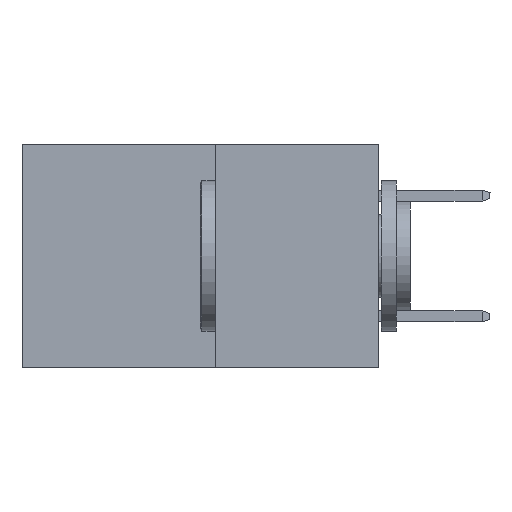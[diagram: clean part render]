
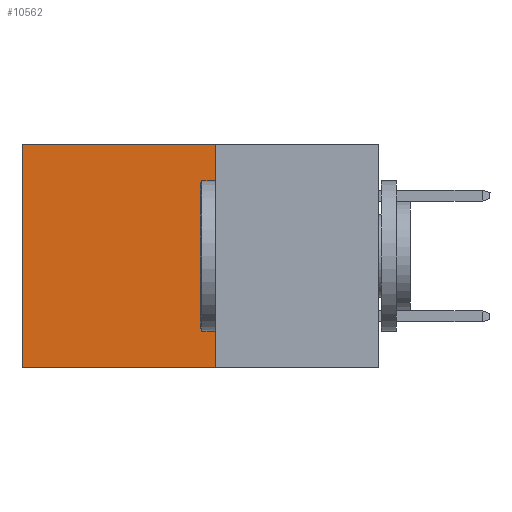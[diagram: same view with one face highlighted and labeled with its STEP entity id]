
A CAD part, left-side view. The second image highlights one B-rep face of the part: STEP entity #10562.
In plain terms, the highlighted planar face has unit normal (-1, 0, 0).
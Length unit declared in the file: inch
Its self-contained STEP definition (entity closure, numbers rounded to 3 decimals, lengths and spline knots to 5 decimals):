
#145 = CARTESIAN_POINT ( 'NONE',  ( 0.277, 0.59, 0. ) ) ;
#256 = EDGE_LOOP ( 'NONE', ( #3795, #10556, #1787, #4095 ) ) ;
#423 = PLANE ( 'NONE',  #4711 ) ;
#491 = CARTESIAN_POINT ( 'NONE',  ( 0.277, 0.27, 0. ) ) ;
#538 = EDGE_CURVE ( 'NONE', #6933, #9746, #675, .T. ) ;
#675 = LINE ( 'NONE', #7138, #7087 ) ;
#751 = VERTEX_POINT ( 'NONE', #6193 ) ;
#1309 = VECTOR ( 'NONE', #8077, 39.37008 ) ;
#1402 = DIRECTION ( 'NONE',  ( 0., 0., -1. ) ) ;
#1787 = ORIENTED_EDGE ( 'NONE', *, *, #4046, .F. ) ;
#3347 = LINE ( 'NONE', #8006, #1309 ) ;
#3415 = FACE_OUTER_BOUND ( 'NONE', #256, .T. ) ;
#3505 = CARTESIAN_POINT ( 'NONE',  ( 0.277, 0.27, -0.37 ) ) ;
#3795 = ORIENTED_EDGE ( 'NONE', *, *, #4185, .T. ) ;
#3926 = CARTESIAN_POINT ( 'NONE',  ( 0.277, 0.59, -0.37 ) ) ;
#4046 = EDGE_CURVE ( 'NONE', #751, #6933, #3347, .T. ) ;
#4095 = ORIENTED_EDGE ( 'NONE', *, *, #9908, .T. ) ;
#4185 = EDGE_CURVE ( 'NONE', #4713, #9746, #4287, .T. ) ;
#4287 = LINE ( 'NONE', #3926, #8557 ) ;
#4711 = AXIS2_PLACEMENT_3D ( 'NONE', #4860, #6624, #1402 ) ;
#4713 = VERTEX_POINT ( 'NONE', #145 ) ;
#4860 = CARTESIAN_POINT ( 'NONE',  ( 0.277, 0.27, -0.37 ) ) ;
#4879 = DIRECTION ( 'NONE',  ( 0., 0., -1. ) ) ;
#4923 = DIRECTION ( 'NONE',  ( 0., 1., 0. ) ) ;
#6193 = CARTESIAN_POINT ( 'NONE',  ( 0.277, 0.27, 0. ) ) ;
#6220 = DIRECTION ( 'NONE',  ( 0., 1., 0. ) ) ;
#6624 = DIRECTION ( 'NONE',  ( 1., 0., 0. ) ) ;
#6832 = VECTOR ( 'NONE', #4923, 39.37008 ) ;
#6933 = VERTEX_POINT ( 'NONE', #3505 ) ;
#7072 = LINE ( 'NONE', #491, #6832 ) ;
#7087 = VECTOR ( 'NONE', #6220, 39.37008 ) ;
#7138 = CARTESIAN_POINT ( 'NONE',  ( 0.277, 0.27, -0.37 ) ) ;
#8006 = CARTESIAN_POINT ( 'NONE',  ( 0.277, 0.27, -0.37 ) ) ;
#8077 = DIRECTION ( 'NONE',  ( 0., 0., -1. ) ) ;
#8115 = CARTESIAN_POINT ( 'NONE',  ( 0.277, 0.59, -0.37 ) ) ;
#8557 = VECTOR ( 'NONE', #4879, 39.37008 ) ;
#9746 = VERTEX_POINT ( 'NONE', #8115 ) ;
#9908 = EDGE_CURVE ( 'NONE', #751, #4713, #7072, .T. ) ;
#10556 = ORIENTED_EDGE ( 'NONE', *, *, #538, .F. ) ;
#10562 = ADVANCED_FACE ( 'NONE', ( #3415 ), #423, .F. ) ;
